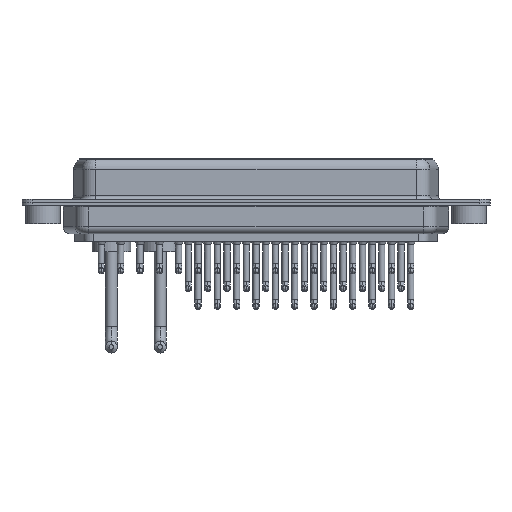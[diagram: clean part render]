
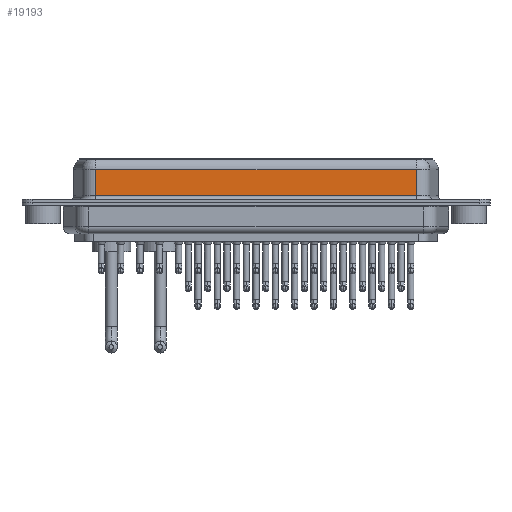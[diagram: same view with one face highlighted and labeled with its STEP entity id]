
A CAD part, front view. The second image highlights one B-rep face of the part: STEP entity #19193.
In plain terms, the highlighted planar face has unit normal (0, -1, 0).
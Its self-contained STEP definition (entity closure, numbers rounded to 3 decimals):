
#2526 = CARTESIAN_POINT ( 'NONE',  ( 7.59, -5.375, 0.9 ) ) ;
#5175 = ORIENTED_EDGE ( 'NONE', *, *, #19044, .T. ) ;
#5923 = DIRECTION ( 'NONE',  ( 0., 0., -1. ) ) ;
#6084 = CARTESIAN_POINT ( 'NONE',  ( 53.41, -5.375, 4.65 ) ) ;
#6957 = VERTEX_POINT ( 'NONE', #22014 ) ;
#7505 = LINE ( 'NONE', #25271, #22791 ) ;
#9538 = EDGE_CURVE ( 'NONE', #32051, #21568, #7505, .T. ) ;
#9603 = LINE ( 'NONE', #31868, #12565 ) ;
#9765 = DIRECTION ( 'NONE',  ( 0., 0., -1. ) ) ;
#10221 = CARTESIAN_POINT ( 'NONE',  ( 53.41, -5.375, 4.65 ) ) ;
#12565 = VECTOR ( 'NONE', #9765, 1000. ) ;
#13285 = AXIS2_PLACEMENT_3D ( 'NONE', #21878, #14469, #24510 ) ;
#13333 = DIRECTION ( 'NONE',  ( -1., 0., 0. ) ) ;
#14297 = FACE_OUTER_BOUND ( 'NONE', #19886, .T. ) ;
#14469 = DIRECTION ( 'NONE',  ( 0., 1., 0. ) ) ;
#18567 = VECTOR ( 'NONE', #13333, 1000. ) ;
#18922 = VERTEX_POINT ( 'NONE', #10221 ) ;
#19044 = EDGE_CURVE ( 'NONE', #18922, #6957, #30827, .T. ) ;
#19193 = ADVANCED_FACE ( 'NONE', ( #14297 ), #24667, .F. ) ;
#19886 = EDGE_LOOP ( 'NONE', ( #23523, #5175, #32529, #26899 ) ) ;
#21547 = LINE ( 'NONE', #26507, #29985 ) ;
#21568 = VERTEX_POINT ( 'NONE', #30740 ) ;
#21878 = CARTESIAN_POINT ( 'NONE',  ( 53.41, -5.375, 6.4 ) ) ;
#22014 = CARTESIAN_POINT ( 'NONE',  ( 7.59, -5.375, 4.65 ) ) ;
#22791 = VECTOR ( 'NONE', #27912, 1000. ) ;
#23523 = ORIENTED_EDGE ( 'NONE', *, *, #24650, .F. ) ;
#24510 = DIRECTION ( 'NONE',  ( 0., 0., 1. ) ) ;
#24650 = EDGE_CURVE ( 'NONE', #18922, #21568, #9603, .T. ) ;
#24667 = PLANE ( 'NONE',  #13285 ) ;
#25271 = CARTESIAN_POINT ( 'NONE',  ( 53.41, -5.375, 0.9 ) ) ;
#26507 = CARTESIAN_POINT ( 'NONE',  ( 7.59, -5.375, 6.4 ) ) ;
#26899 = ORIENTED_EDGE ( 'NONE', *, *, #9538, .T. ) ;
#27912 = DIRECTION ( 'NONE',  ( 1., 0., 0. ) ) ;
#28117 = EDGE_CURVE ( 'NONE', #6957, #32051, #21547, .T. ) ;
#29985 = VECTOR ( 'NONE', #5923, 1000. ) ;
#30740 = CARTESIAN_POINT ( 'NONE',  ( 53.41, -5.375, 0.9 ) ) ;
#30827 = LINE ( 'NONE', #6084, #18567 ) ;
#31868 = CARTESIAN_POINT ( 'NONE',  ( 53.41, -5.375, 6.4 ) ) ;
#32051 = VERTEX_POINT ( 'NONE', #2526 ) ;
#32529 = ORIENTED_EDGE ( 'NONE', *, *, #28117, .T. ) ;
